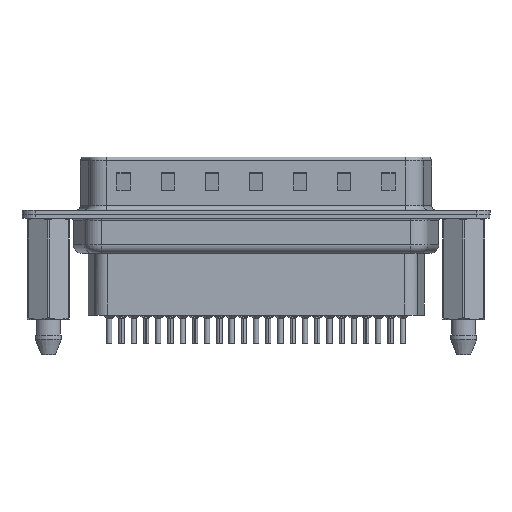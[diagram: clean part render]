
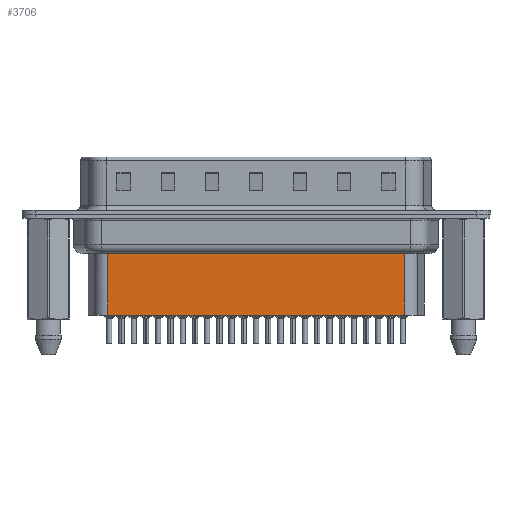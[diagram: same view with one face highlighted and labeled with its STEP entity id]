
A CAD part, front view. The second image highlights one B-rep face of the part: STEP entity #3706.
In plain terms, the highlighted planar face has unit normal (0, -1, 0).
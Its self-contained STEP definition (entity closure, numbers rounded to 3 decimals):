
#1024 = CARTESIAN_POINT ( 'NONE',  ( 40.344, -3.5, -11.45 ) ) ;
#2498 = ORIENTED_EDGE ( 'NONE', *, *, #27771, .T. ) ;
#2876 = LINE ( 'NONE', #16300, #19384 ) ;
#3706 = ADVANCED_FACE ( 'NONE', ( #26107 ), #21101, .T. ) ;
#4951 = CARTESIAN_POINT ( 'NONE',  ( 6.459, -3.5, -4.097 ) ) ;
#5301 = LINE ( 'NONE', #21637, #27438 ) ;
#5939 = ORIENTED_EDGE ( 'NONE', *, *, #21962, .F. ) ;
#7421 = VERTEX_POINT ( 'NONE', #1024 ) ;
#8843 = CARTESIAN_POINT ( 'NONE',  ( 6.706, -3.5, -11.45 ) ) ;
#8867 = DIRECTION ( 'NONE',  ( -1., 0., 0. ) ) ;
#9938 = DIRECTION ( 'NONE',  ( 0., 0., -1. ) ) ;
#10768 = VECTOR ( 'NONE', #19992, 1000. ) ;
#12036 = CARTESIAN_POINT ( 'NONE',  ( 6.706, -3.5, -3.1 ) ) ;
#12209 = CARTESIAN_POINT ( 'NONE',  ( 40.344, -3.5, -4.097 ) ) ;
#12896 = CARTESIAN_POINT ( 'NONE',  ( 6.706, -3.5, -4.097 ) ) ;
#13106 = EDGE_CURVE ( 'NONE', #7421, #13780, #5301, .T. ) ;
#13780 = VERTEX_POINT ( 'NONE', #8843 ) ;
#14110 = EDGE_CURVE ( 'NONE', #15912, #13780, #19780, .T. ) ;
#14112 = VECTOR ( 'NONE', #9938, 1000. ) ;
#15014 = ORIENTED_EDGE ( 'NONE', *, *, #14110, .T. ) ;
#15360 = AXIS2_PLACEMENT_3D ( 'NONE', #24921, #22789, #22769 ) ;
#15912 = VERTEX_POINT ( 'NONE', #12896 ) ;
#16300 = CARTESIAN_POINT ( 'NONE',  ( 40.344, -3.5, -3.1 ) ) ;
#18378 = ORIENTED_EDGE ( 'NONE', *, *, #13106, .F. ) ;
#18809 = EDGE_LOOP ( 'NONE', ( #5939, #2498, #15014, #18378 ) ) ;
#19384 = VECTOR ( 'NONE', #20586, 1000. ) ;
#19780 = LINE ( 'NONE', #12036, #14112 ) ;
#19992 = DIRECTION ( 'NONE',  ( -1., 0., 0. ) ) ;
#20586 = DIRECTION ( 'NONE',  ( 0., 0., -1. ) ) ;
#21101 = PLANE ( 'NONE',  #15360 ) ;
#21637 = CARTESIAN_POINT ( 'NONE',  ( 6.706, -3.5, -11.45 ) ) ;
#21962 = EDGE_CURVE ( 'NONE', #22815, #7421, #2876, .T. ) ;
#22081 = LINE ( 'NONE', #4951, #10768 ) ;
#22769 = DIRECTION ( 'NONE',  ( 1., 0., 0. ) ) ;
#22789 = DIRECTION ( 'NONE',  ( 0., -1., 0. ) ) ;
#22815 = VERTEX_POINT ( 'NONE', #12209 ) ;
#24921 = CARTESIAN_POINT ( 'NONE',  ( 6.706, -3.5, -3.1 ) ) ;
#26107 = FACE_OUTER_BOUND ( 'NONE', #18809, .T. ) ;
#27438 = VECTOR ( 'NONE', #8867, 1000. ) ;
#27771 = EDGE_CURVE ( 'NONE', #22815, #15912, #22081, .T. ) ;
